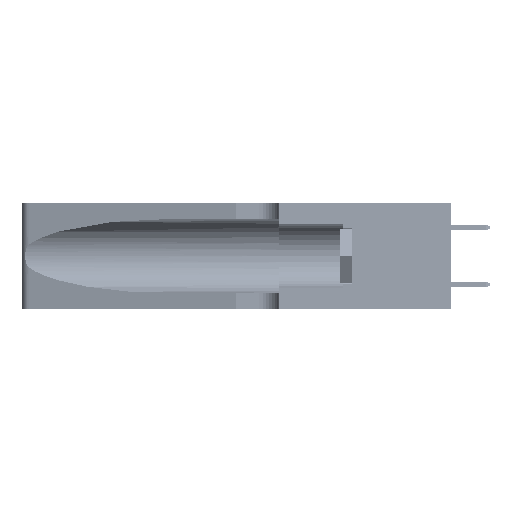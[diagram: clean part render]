
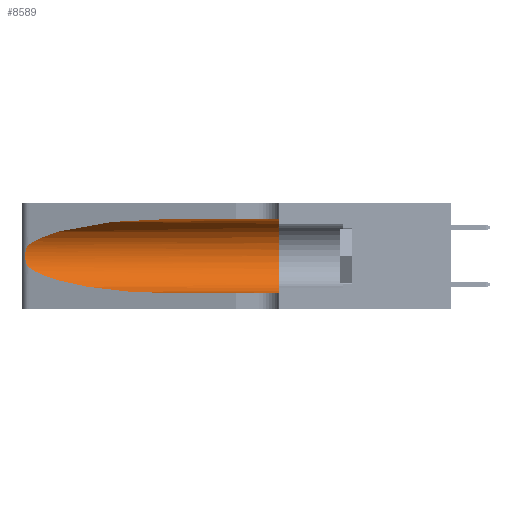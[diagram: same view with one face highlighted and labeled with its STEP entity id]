
A CAD part, left-side view. The second image highlights one B-rep face of the part: STEP entity #8589.
In plain terms, the highlighted cylindrical face has radius 3.308 mm (diameter 6.617 mm), a partial arc.
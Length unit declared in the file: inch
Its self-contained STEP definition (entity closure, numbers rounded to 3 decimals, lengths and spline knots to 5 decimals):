
#416 = EDGE_LOOP ( 'NONE', ( #48100, #3165, #38986, #39955, #40630, #41513 ) ) ;
#838 = B_SPLINE_CURVE_WITH_KNOTS ( 'NONE', 3,
 ( #36632, #1436, #29312, #1953, #12896, #17849, #28795, #916, #29042, #13151, #9756, #33761, #16819, #33511 ),
 .UNSPECIFIED., .F., .F.,
 ( 4, 2, 2, 2, 2, 2, 4 ),
 ( 0., 0.00027, 0.00053, 0.00107, 0.0016, 0.00187, 0.00214 ),
 .UNSPECIFIED. ) ;
#916 = CARTESIAN_POINT ( 'NONE',  ( 0.26075, 1.23896, 0.178 ) ) ;
#1259 = CARTESIAN_POINT ( 'NONE',  ( 0.18966, 0.96281, 0.05475 ) ) ;
#1436 = CARTESIAN_POINT ( 'NONE',  ( 0.25555, 1.22994, 0.2215 ) ) ;
#1860 = CARTESIAN_POINT ( 'NONE',  ( 0.1305, 0.35, 0.05475 ) ) ;
#1953 = CARTESIAN_POINT ( 'NONE',  ( 0.25787, 1.23484, 0.2124 ) ) ;
#2420 = VERTEX_POINT ( 'NONE', #16872 ) ;
#2774 = CARTESIAN_POINT ( 'NONE',  ( 0.1305, 0.72297, 0.05475 ) ) ;
#3165 = ORIENTED_EDGE ( 'NONE', *, *, #18902, .T. ) ;
#4123 =( BOUNDED_CURVE ( )  B_SPLINE_CURVE ( 3, ( #40866, #21044, #1259, #38016 ),
 .UNSPECIFIED., .F., .T. ) 
 B_SPLINE_CURVE_WITH_KNOTS ( ( 4, 4 ),
 ( 3.44316, 4.71239 ),
 .UNSPECIFIED. ) 
 CURVE ( )  GEOMETRIC_REPRESENTATION_ITEM ( )  RATIONAL_B_SPLINE_CURVE ( ( 1., 0.87, 0.87, 1. ) ) 
 REPRESENTATION_ITEM ( '' )  );
#4533 = DIRECTION ( 'NONE',  ( 0., 0., -1. ) ) ;
#5176 = VECTOR ( 'NONE', #41794, 39.37008 ) ;
#6490 = CARTESIAN_POINT ( 'NONE',  ( 0.2373, 1.15595, 0.28018 ) ) ;
#6600 = LINE ( 'NONE', #50888, #5176 ) ;
#8589 = ADVANCED_FACE ( 'NONE', ( #12841 ), #36341, .F. ) ;
#9756 = CARTESIAN_POINT ( 'NONE',  ( 0.25789, 1.23486, 0.15765 ) ) ;
#12335 = CARTESIAN_POINT ( 'NONE',  ( 0.1305, 1.61858, 0.185 ) ) ;
#12561 = CARTESIAN_POINT ( 'NONE',  ( 0.1305, 0.35, 0.185 ) ) ;
#12841 = FACE_OUTER_BOUND ( 'NONE', #416, .T. ) ;
#12896 = CARTESIAN_POINT ( 'NONE',  ( 0.25854, 1.2359, 0.20912 ) ) ;
#13151 = CARTESIAN_POINT ( 'NONE',  ( 0.25856, 1.23593, 0.16098 ) ) ;
#15063 = VERTEX_POINT ( 'NONE', #33126 ) ;
#16173 = CARTESIAN_POINT ( 'NONE',  ( 0.1305, 0.72297, 0.31525 ) ) ;
#16819 = CARTESIAN_POINT ( 'NONE',  ( 0.25555, 1.22993, 0.14849 ) ) ;
#16872 = CARTESIAN_POINT ( 'NONE',  ( 0.25487, 1.22718, 0.14631 ) ) ;
#17849 = CARTESIAN_POINT ( 'NONE',  ( 0.26018, 1.23835, 0.19895 ) ) ;
#18371 = CIRCLE ( 'NONE', #33363, 0.13025 ) ;
#18902 = EDGE_CURVE ( 'NONE', #15063, #2420, #838, .T. ) ;
#20544 = AXIS2_PLACEMENT_3D ( 'NONE', #12335, #40249, #4533 ) ;
#20829 = EDGE_CURVE ( 'NONE', #42407, #28715, #6600, .T. ) ;
#21044 = CARTESIAN_POINT ( 'NONE',  ( 0.2373, 1.15595, 0.08982 ) ) ;
#23539 = EDGE_CURVE ( 'NONE', #2420, #30361, #4123, .T. ) ;
#24294 = DIRECTION ( 'NONE',  ( 0., 1., 0. ) ) ;
#25168 = CARTESIAN_POINT ( 'NONE',  ( 0.1305, 1.61858, 0.05475 ) ) ;
#27124 =( BOUNDED_CURVE ( )  B_SPLINE_CURVE ( 3, ( #34646, #27307, #6490, #43211 ),
 .UNSPECIFIED., .F., .T. ) 
 B_SPLINE_CURVE_WITH_KNOTS ( ( 4, 4 ),
 ( 1.5708, 2.84003 ),
 .UNSPECIFIED. ) 
 CURVE ( )  GEOMETRIC_REPRESENTATION_ITEM ( )  RATIONAL_B_SPLINE_CURVE ( ( 1., 0.87, 0.87, 1. ) ) 
 REPRESENTATION_ITEM ( '' )  );
#27307 = CARTESIAN_POINT ( 'NONE',  ( 0.18966, 0.96281, 0.31525 ) ) ;
#28715 = VERTEX_POINT ( 'NONE', #46400 ) ;
#28795 = CARTESIAN_POINT ( 'NONE',  ( 0.26075, 1.23896, 0.19203 ) ) ;
#29042 = CARTESIAN_POINT ( 'NONE',  ( 0.26017, 1.23833, 0.17102 ) ) ;
#29312 = CARTESIAN_POINT ( 'NONE',  ( 0.25639, 1.23184, 0.21858 ) ) ;
#29342 = LINE ( 'NONE', #25168, #51426 ) ;
#29452 = EDGE_CURVE ( 'NONE', #30361, #44729, #29342, .T. ) ;
#29599 = DIRECTION ( 'NONE',  ( 0., -1., 0. ) ) ;
#30361 = VERTEX_POINT ( 'NONE', #2774 ) ;
#32390 = EDGE_CURVE ( 'NONE', #28715, #44729, #18371, .T. ) ;
#33126 = CARTESIAN_POINT ( 'NONE',  ( 0.25487, 1.22718, 0.22369 ) ) ;
#33363 = AXIS2_PLACEMENT_3D ( 'NONE', #12561, #24294, #48276 ) ;
#33511 = CARTESIAN_POINT ( 'NONE',  ( 0.25487, 1.22718, 0.14631 ) ) ;
#33761 = CARTESIAN_POINT ( 'NONE',  ( 0.25639, 1.23186, 0.15144 ) ) ;
#34646 = CARTESIAN_POINT ( 'NONE',  ( 0.1305, 0.72297, 0.31525 ) ) ;
#36341 = CYLINDRICAL_SURFACE ( 'NONE', #20544, 0.13025 ) ;
#36632 = CARTESIAN_POINT ( 'NONE',  ( 0.25487, 1.22718, 0.22369 ) ) ;
#38016 = CARTESIAN_POINT ( 'NONE',  ( 0.1305, 0.72297, 0.05475 ) ) ;
#38986 = ORIENTED_EDGE ( 'NONE', *, *, #23539, .T. ) ;
#39955 = ORIENTED_EDGE ( 'NONE', *, *, #29452, .T. ) ;
#40249 = DIRECTION ( 'NONE',  ( 0., -1., 0. ) ) ;
#40630 = ORIENTED_EDGE ( 'NONE', *, *, #32390, .F. ) ;
#40866 = CARTESIAN_POINT ( 'NONE',  ( 0.25487, 1.22718, 0.14631 ) ) ;
#41513 = ORIENTED_EDGE ( 'NONE', *, *, #20829, .F. ) ;
#41794 = DIRECTION ( 'NONE',  ( 0., -1., 0. ) ) ;
#42407 = VERTEX_POINT ( 'NONE', #16173 ) ;
#43211 = CARTESIAN_POINT ( 'NONE',  ( 0.25487, 1.22718, 0.22369 ) ) ;
#43921 = EDGE_CURVE ( 'NONE', #42407, #15063, #27124, .T. ) ;
#44729 = VERTEX_POINT ( 'NONE', #1860 ) ;
#46400 = CARTESIAN_POINT ( 'NONE',  ( 0.1305, 0.35, 0.31525 ) ) ;
#48100 = ORIENTED_EDGE ( 'NONE', *, *, #43921, .T. ) ;
#48276 = DIRECTION ( 'NONE',  ( 0., 0., 1. ) ) ;
#50888 = CARTESIAN_POINT ( 'NONE',  ( 0.1305, 1.61858, 0.31525 ) ) ;
#51426 = VECTOR ( 'NONE', #29599, 39.37008 ) ;
